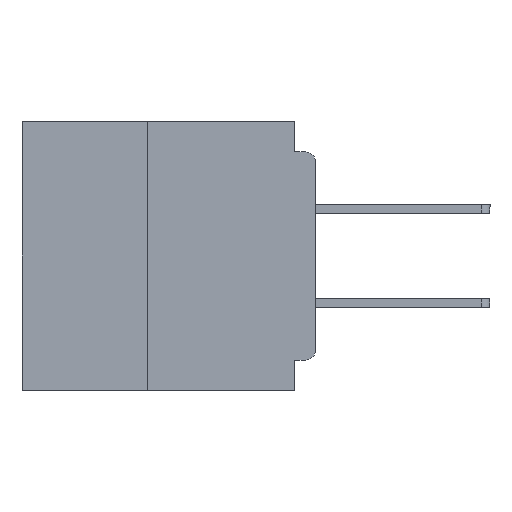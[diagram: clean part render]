
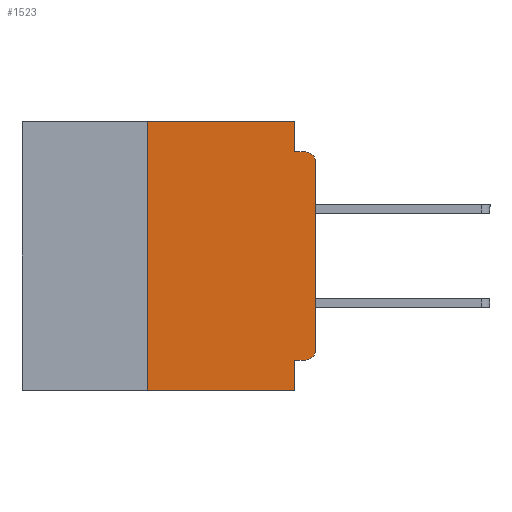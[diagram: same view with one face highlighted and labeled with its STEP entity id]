
A CAD part, left-side view. The second image highlights one B-rep face of the part: STEP entity #1523.
In plain terms, the highlighted planar face has unit normal (-1, 0, 0).
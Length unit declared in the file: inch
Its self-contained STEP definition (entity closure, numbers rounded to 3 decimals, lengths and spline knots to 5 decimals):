
#792 = VERTEX_POINT ( 'NONE', #33663 ) ;
#895 = VECTOR ( 'NONE', #24722, 39.37008 ) ;
#1523 = ADVANCED_FACE ( 'NONE', ( #15305 ), #8143, .F. ) ;
#2361 = ORIENTED_EDGE ( 'NONE', *, *, #35334, .T. ) ;
#2426 = VERTEX_POINT ( 'NONE', #4041 ) ;
#2681 = VERTEX_POINT ( 'NONE', #24352 ) ;
#3008 = CARTESIAN_POINT ( 'NONE',  ( 0., 0.031, -0.4 ) ) ;
#3526 = CARTESIAN_POINT ( 'NONE',  ( 0., 0., -0.045 ) ) ;
#3752 = DIRECTION ( 'NONE',  ( 0., 0., -1. ) ) ;
#3792 = DIRECTION ( 'NONE',  ( -1., 0., 0. ) ) ;
#3839 = CARTESIAN_POINT ( 'NONE',  ( 0., 0.015, -0.06 ) ) ;
#3984 = DIRECTION ( 'NONE',  ( 0., 0., 1. ) ) ;
#4010 = CARTESIAN_POINT ( 'NONE',  ( 0., 0.031, 0. ) ) ;
#4041 = CARTESIAN_POINT ( 'NONE',  ( 0., 0.015, -0.045 ) ) ;
#4282 = ORIENTED_EDGE ( 'NONE', *, *, #6025, .T. ) ;
#4971 = LINE ( 'NONE', #21222, #19260 ) ;
#5618 = VERTEX_POINT ( 'NONE', #12185 ) ;
#6025 = EDGE_CURVE ( 'NONE', #24868, #2426, #22683, .T. ) ;
#6115 = DIRECTION ( 'NONE',  ( 0., 0., -1. ) ) ;
#6150 = LINE ( 'NONE', #4010, #35274 ) ;
#6210 = ORIENTED_EDGE ( 'NONE', *, *, #13898, .F. ) ;
#7723 = EDGE_CURVE ( 'NONE', #32089, #13083, #4971, .T. ) ;
#8143 = PLANE ( 'NONE',  #21613 ) ;
#8224 = CARTESIAN_POINT ( 'NONE',  ( 0., 0.437, 0. ) ) ;
#9152 = EDGE_CURVE ( 'NONE', #28762, #13083, #32219, .T. ) ;
#9746 = CIRCLE ( 'NONE', #23490, 0.015 ) ;
#10970 = LINE ( 'NONE', #25187, #17125 ) ;
#11239 = CARTESIAN_POINT ( 'NONE',  ( 0., 0.437, 0. ) ) ;
#11270 = EDGE_CURVE ( 'NONE', #2681, #2426, #15247, .T. ) ;
#11380 = VERTEX_POINT ( 'NONE', #36987 ) ;
#11632 = CARTESIAN_POINT ( 'NONE',  ( 0., 0.031, -0.4 ) ) ;
#12175 = EDGE_CURVE ( 'NONE', #792, #28762, #30177, .T. ) ;
#12185 = CARTESIAN_POINT ( 'NONE',  ( 0., 0.031, 0. ) ) ;
#12973 = DIRECTION ( 'NONE',  ( -1., 0., 0. ) ) ;
#13083 = VERTEX_POINT ( 'NONE', #3008 ) ;
#13898 = EDGE_CURVE ( 'NONE', #5618, #2681, #6150, .T. ) ;
#14266 = DIRECTION ( 'NONE',  ( 0., -1., 0. ) ) ;
#15247 = LINE ( 'NONE', #3526, #895 ) ;
#15305 = FACE_OUTER_BOUND ( 'NONE', #17860, .T. ) ;
#16578 = CARTESIAN_POINT ( 'NONE',  ( 0., 0.25, 0. ) ) ;
#17125 = VECTOR ( 'NONE', #3984, 39.37008 ) ;
#17294 = DIRECTION ( 'NONE',  ( 0., 0., 1. ) ) ;
#17860 = EDGE_LOOP ( 'NONE', ( #2361, #4282, #20477, #6210, #33578, #28525, #36328, #30373, #23364, #26188 ) ) ;
#19260 = VECTOR ( 'NONE', #21229, 39.37008 ) ;
#20477 = ORIENTED_EDGE ( 'NONE', *, *, #11270, .F. ) ;
#21222 = CARTESIAN_POINT ( 'NONE',  ( 0., 0.437, -0.4 ) ) ;
#21229 = DIRECTION ( 'NONE',  ( 0., -1., 0. ) ) ;
#21613 = AXIS2_PLACEMENT_3D ( 'NONE', #8224, #26242, #6115 ) ;
#22683 = CIRCLE ( 'NONE', #25203, 0.015 ) ;
#23047 = LINE ( 'NONE', #38059, #38754 ) ;
#23364 = ORIENTED_EDGE ( 'NONE', *, *, #12175, .F. ) ;
#23490 = AXIS2_PLACEMENT_3D ( 'NONE', #30956, #12973, #33884 ) ;
#23567 = LINE ( 'NONE', #11239, #30574 ) ;
#24352 = CARTESIAN_POINT ( 'NONE',  ( 0., 0.031, -0.045 ) ) ;
#24558 = EDGE_CURVE ( 'NONE', #28937, #5618, #23567, .T. ) ;
#24655 = CARTESIAN_POINT ( 'NONE',  ( 0., 0., -0.06 ) ) ;
#24722 = DIRECTION ( 'NONE',  ( 0., -1., 0. ) ) ;
#24868 = VERTEX_POINT ( 'NONE', #24655 ) ;
#25187 = CARTESIAN_POINT ( 'NONE',  ( 0., 0., 0. ) ) ;
#25203 = AXIS2_PLACEMENT_3D ( 'NONE', #3839, #3792, #3752 ) ;
#25226 = EDGE_CURVE ( 'NONE', #32089, #28937, #23047, .T. ) ;
#26063 = CARTESIAN_POINT ( 'NONE',  ( 0., 0.25, -0.4 ) ) ;
#26188 = ORIENTED_EDGE ( 'NONE', *, *, #33006, .T. ) ;
#26242 = DIRECTION ( 'NONE',  ( 1., 0., 0. ) ) ;
#28525 = ORIENTED_EDGE ( 'NONE', *, *, #25226, .F. ) ;
#28762 = VERTEX_POINT ( 'NONE', #36622 ) ;
#28937 = VERTEX_POINT ( 'NONE', #16578 ) ;
#29255 = VECTOR ( 'NONE', #38219, 39.37008 ) ;
#30177 = LINE ( 'NONE', #35280, #29255 ) ;
#30373 = ORIENTED_EDGE ( 'NONE', *, *, #9152, .F. ) ;
#30574 = VECTOR ( 'NONE', #14266, 39.37008 ) ;
#30956 = CARTESIAN_POINT ( 'NONE',  ( 0., 0.015, -0.34 ) ) ;
#31198 = DIRECTION ( 'NONE',  ( 0., 0., -1. ) ) ;
#31294 = VECTOR ( 'NONE', #35539, 39.37008 ) ;
#32089 = VERTEX_POINT ( 'NONE', #26063 ) ;
#32219 = LINE ( 'NONE', #11632, #31294 ) ;
#33006 = EDGE_CURVE ( 'NONE', #792, #11380, #9746, .T. ) ;
#33578 = ORIENTED_EDGE ( 'NONE', *, *, #24558, .F. ) ;
#33663 = CARTESIAN_POINT ( 'NONE',  ( 0., 0.015, -0.355 ) ) ;
#33884 = DIRECTION ( 'NONE',  ( 0., 0., -1. ) ) ;
#35274 = VECTOR ( 'NONE', #31198, 39.37008 ) ;
#35280 = CARTESIAN_POINT ( 'NONE',  ( 0., 0., -0.355 ) ) ;
#35334 = EDGE_CURVE ( 'NONE', #11380, #24868, #10970, .T. ) ;
#35539 = DIRECTION ( 'NONE',  ( 0., 0., -1. ) ) ;
#36328 = ORIENTED_EDGE ( 'NONE', *, *, #7723, .T. ) ;
#36622 = CARTESIAN_POINT ( 'NONE',  ( 0., 0.031, -0.355 ) ) ;
#36987 = CARTESIAN_POINT ( 'NONE',  ( 0., 0., -0.34 ) ) ;
#38059 = CARTESIAN_POINT ( 'NONE',  ( 0., 0.25, -0.4 ) ) ;
#38219 = DIRECTION ( 'NONE',  ( 0., 1., 0. ) ) ;
#38754 = VECTOR ( 'NONE', #17294, 39.37008 ) ;
